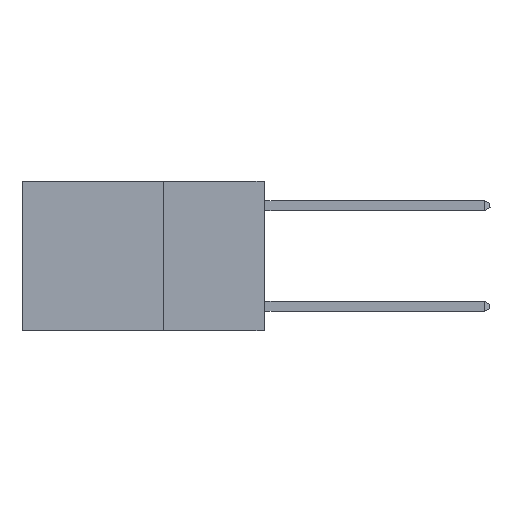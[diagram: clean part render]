
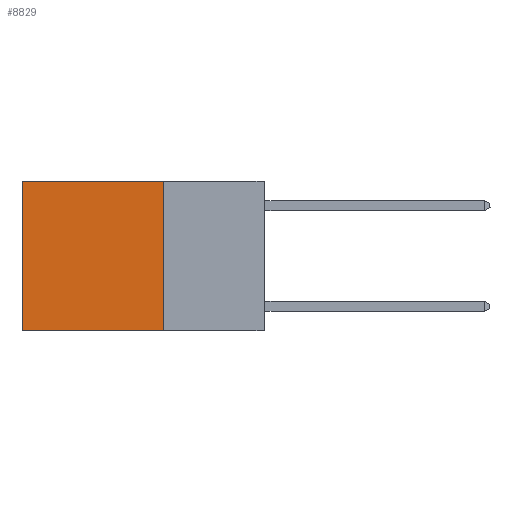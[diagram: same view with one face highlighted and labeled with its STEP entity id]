
A CAD part, left-side view. The second image highlights one B-rep face of the part: STEP entity #8829.
In plain terms, the highlighted planar face has unit normal (-1, 0, 0).
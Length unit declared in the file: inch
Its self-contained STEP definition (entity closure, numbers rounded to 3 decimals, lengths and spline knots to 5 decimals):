
#1747 = VERTEX_POINT ( 'NONE', #1868 ) ;
#1840 = CARTESIAN_POINT ( 'NONE',  ( 0.2625, 0.6, 0. ) ) ;
#1868 = CARTESIAN_POINT ( 'NONE',  ( 0.2625, 0.6, -0.37 ) ) ;
#2060 = EDGE_LOOP ( 'NONE', ( #14218, #18700, #11121, #15585 ) ) ;
#3881 = AXIS2_PLACEMENT_3D ( 'NONE', #17898, #13131, #30019 ) ;
#4010 = CARTESIAN_POINT ( 'NONE',  ( 0.2625, 0.25, -0.37 ) ) ;
#8273 = VERTEX_POINT ( 'NONE', #4010 ) ;
#8500 = LINE ( 'NONE', #19403, #26984 ) ;
#8829 = ADVANCED_FACE ( 'NONE', ( #22882 ), #25139, .F. ) ;
#8917 = CARTESIAN_POINT ( 'NONE',  ( 0.2625, 0.25, 0. ) ) ;
#9426 = VECTOR ( 'NONE', #13241, 39.37008 ) ;
#9458 = EDGE_CURVE ( 'NONE', #8273, #1747, #25440, .T. ) ;
#11121 = ORIENTED_EDGE ( 'NONE', *, *, #19090, .F. ) ;
#12625 = VECTOR ( 'NONE', #15043, 39.37008 ) ;
#13131 = DIRECTION ( 'NONE',  ( 1., 0., 0. ) ) ;
#13241 = DIRECTION ( 'NONE',  ( 0., 0., -1. ) ) ;
#13345 = CARTESIAN_POINT ( 'NONE',  ( 0.2625, 0.6, 0. ) ) ;
#14218 = ORIENTED_EDGE ( 'NONE', *, *, #26852, .T. ) ;
#15043 = DIRECTION ( 'NONE',  ( 0., 1., 0. ) ) ;
#15585 = ORIENTED_EDGE ( 'NONE', *, *, #21509, .T. ) ;
#15868 = LINE ( 'NONE', #13345, #9426 ) ;
#16134 = DIRECTION ( 'NONE',  ( 0., 1., 0. ) ) ;
#17898 = CARTESIAN_POINT ( 'NONE',  ( 0.2625, 0.25, 0. ) ) ;
#18202 = CARTESIAN_POINT ( 'NONE',  ( 0.2625, 0.25, 0. ) ) ;
#18700 = ORIENTED_EDGE ( 'NONE', *, *, #9458, .F. ) ;
#19090 = EDGE_CURVE ( 'NONE', #24042, #8273, #8500, .T. ) ;
#19403 = CARTESIAN_POINT ( 'NONE',  ( 0.2625, 0.25, 0. ) ) ;
#20138 = LINE ( 'NONE', #8917, #25008 ) ;
#21509 = EDGE_CURVE ( 'NONE', #24042, #24200, #20138, .T. ) ;
#21733 = DIRECTION ( 'NONE',  ( 0., 0., -1. ) ) ;
#22882 = FACE_OUTER_BOUND ( 'NONE', #2060, .T. ) ;
#24042 = VERTEX_POINT ( 'NONE', #18202 ) ;
#24200 = VERTEX_POINT ( 'NONE', #1840 ) ;
#25008 = VECTOR ( 'NONE', #16134, 39.37008 ) ;
#25139 = PLANE ( 'NONE',  #3881 ) ;
#25440 = LINE ( 'NONE', #29480, #12625 ) ;
#26852 = EDGE_CURVE ( 'NONE', #24200, #1747, #15868, .T. ) ;
#26984 = VECTOR ( 'NONE', #21733, 39.37008 ) ;
#29480 = CARTESIAN_POINT ( 'NONE',  ( 0.2625, 0.25, -0.37 ) ) ;
#30019 = DIRECTION ( 'NONE',  ( 0., 0., -1. ) ) ;
